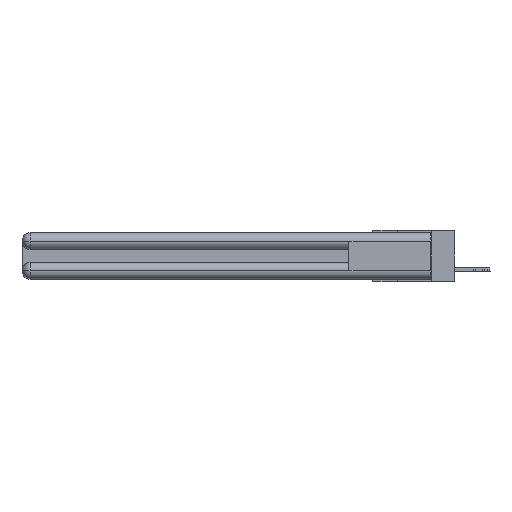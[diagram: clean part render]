
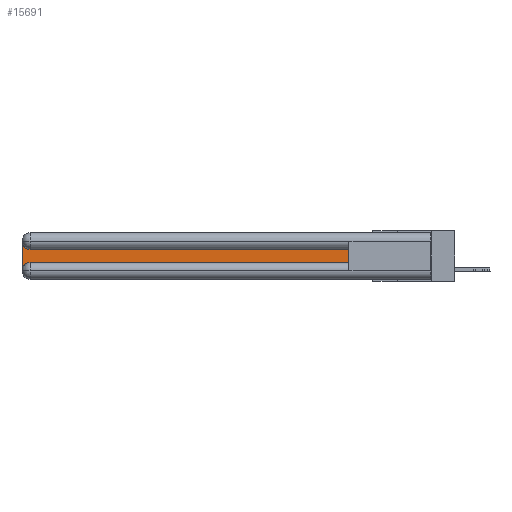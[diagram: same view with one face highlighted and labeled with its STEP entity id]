
A CAD part, left-side view. The second image highlights one B-rep face of the part: STEP entity #15691.
In plain terms, the highlighted planar face has unit normal (-1, 0, 0).
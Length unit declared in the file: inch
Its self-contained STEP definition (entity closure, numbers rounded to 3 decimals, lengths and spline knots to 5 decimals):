
#747 = CARTESIAN_POINT ( 'NONE',  ( 0.075, 0.6, -0.1225 ) ) ;
#1322 = EDGE_CURVE ( 'NONE', #27611, #8026, #6199, .T. ) ;
#1616 = CARTESIAN_POINT ( 'NONE',  ( 0.075, 0.6, -0.1225 ) ) ;
#1716 = CARTESIAN_POINT ( 'NONE',  ( 0.075, 3., -0.0625 ) ) ;
#2591 = CARTESIAN_POINT ( 'NONE',  ( 0.075, 2.94, -0.2775 ) ) ;
#2802 = VECTOR ( 'NONE', #15602, 39.37008 ) ;
#2987 = EDGE_LOOP ( 'NONE', ( #24105, #28590, #6815, #17760, #16028, #3757 ) ) ;
#3223 = CIRCLE ( 'NONE', #11296, 0.06 ) ;
#3429 = VERTEX_POINT ( 'NONE', #5814 ) ;
#3757 = ORIENTED_EDGE ( 'NONE', *, *, #1322, .T. ) ;
#3776 = EDGE_CURVE ( 'NONE', #16320, #22658, #24422, .T. ) ;
#5111 = AXIS2_PLACEMENT_3D ( 'NONE', #16882, #12152, #28506 ) ;
#5814 = CARTESIAN_POINT ( 'NONE',  ( 0.075, 2.94, -0.1225 ) ) ;
#6121 = CARTESIAN_POINT ( 'NONE',  ( 0.075, 3., -0.1225 ) ) ;
#6177 = DIRECTION ( 'NONE',  ( 0., 0., 1. ) ) ;
#6199 = LINE ( 'NONE', #20151, #15679 ) ;
#6363 = CARTESIAN_POINT ( 'NONE',  ( 0.075, 3., -0.2775 ) ) ;
#6815 = ORIENTED_EDGE ( 'NONE', *, *, #3776, .T. ) ;
#7494 = CARTESIAN_POINT ( 'NONE',  ( 0.075, 2.94, -0.2175 ) ) ;
#8026 = VERTEX_POINT ( 'NONE', #747 ) ;
#8435 = DIRECTION ( 'NONE',  ( 1., 0., 0. ) ) ;
#8542 = PLANE ( 'NONE',  #27023 ) ;
#9894 = LINE ( 'NONE', #12342, #13578 ) ;
#10000 = VERTEX_POINT ( 'NONE', #7494 ) ;
#11296 = AXIS2_PLACEMENT_3D ( 'NONE', #2591, #19014, #14323 ) ;
#12152 = DIRECTION ( 'NONE',  ( 1., 0., 0. ) ) ;
#12342 = CARTESIAN_POINT ( 'NONE',  ( 0.075, 0.6, -0.2175 ) ) ;
#13402 = EDGE_CURVE ( 'NONE', #22658, #10000, #3223, .T. ) ;
#13578 = VECTOR ( 'NONE', #28358, 39.37008 ) ;
#14323 = DIRECTION ( 'NONE',  ( 0., 0., -1. ) ) ;
#14680 = FACE_OUTER_BOUND ( 'NONE', #2987, .T. ) ;
#15225 = LINE ( 'NONE', #1616, #2802 ) ;
#15235 = DIRECTION ( 'NONE',  ( 0., 0., -1. ) ) ;
#15602 = DIRECTION ( 'NONE',  ( 0., 1., 0. ) ) ;
#15679 = VECTOR ( 'NONE', #6177, 39.37008 ) ;
#15691 = ADVANCED_FACE ( 'NONE', ( #14680 ), #8542, .F. ) ;
#16028 = ORIENTED_EDGE ( 'NONE', *, *, #16194, .T. ) ;
#16194 = EDGE_CURVE ( 'NONE', #10000, #27611, #9894, .T. ) ;
#16320 = VERTEX_POINT ( 'NONE', #1716 ) ;
#16882 = CARTESIAN_POINT ( 'NONE',  ( 0.075, 2.94, -0.0625 ) ) ;
#17760 = ORIENTED_EDGE ( 'NONE', *, *, #13402, .T. ) ;
#19014 = DIRECTION ( 'NONE',  ( 1., 0., 0. ) ) ;
#19408 = EDGE_CURVE ( 'NONE', #8026, #3429, #15225, .T. ) ;
#20151 = CARTESIAN_POINT ( 'NONE',  ( 0.075, 0.6, -0.2175 ) ) ;
#22210 = VECTOR ( 'NONE', #15235, 39.37008 ) ;
#22458 = DIRECTION ( 'NONE',  ( 0., 0., -1. ) ) ;
#22658 = VERTEX_POINT ( 'NONE', #6363 ) ;
#24105 = ORIENTED_EDGE ( 'NONE', *, *, #19408, .T. ) ;
#24422 = LINE ( 'NONE', #26676, #22210 ) ;
#24528 = CARTESIAN_POINT ( 'NONE',  ( 0.075, 0.6, -0.2175 ) ) ;
#26417 = CIRCLE ( 'NONE', #5111, 0.06 ) ;
#26676 = CARTESIAN_POINT ( 'NONE',  ( 0.075, 3., -0.2175 ) ) ;
#27023 = AXIS2_PLACEMENT_3D ( 'NONE', #6121, #8435, #22458 ) ;
#27611 = VERTEX_POINT ( 'NONE', #24528 ) ;
#28358 = DIRECTION ( 'NONE',  ( 0., -1., 0. ) ) ;
#28506 = DIRECTION ( 'NONE',  ( 0., 0., -1. ) ) ;
#28590 = ORIENTED_EDGE ( 'NONE', *, *, #30246, .T. ) ;
#30246 = EDGE_CURVE ( 'NONE', #3429, #16320, #26417, .T. ) ;
